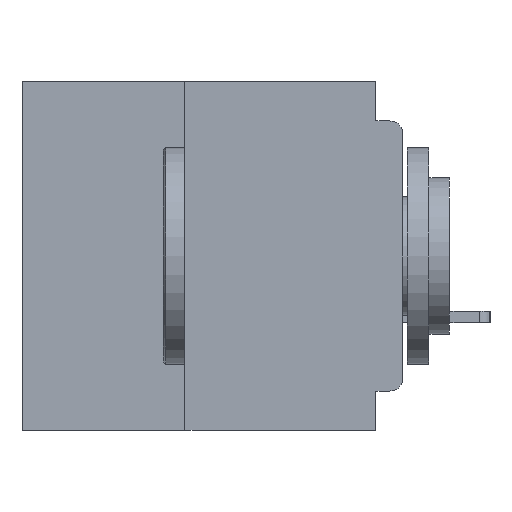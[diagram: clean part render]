
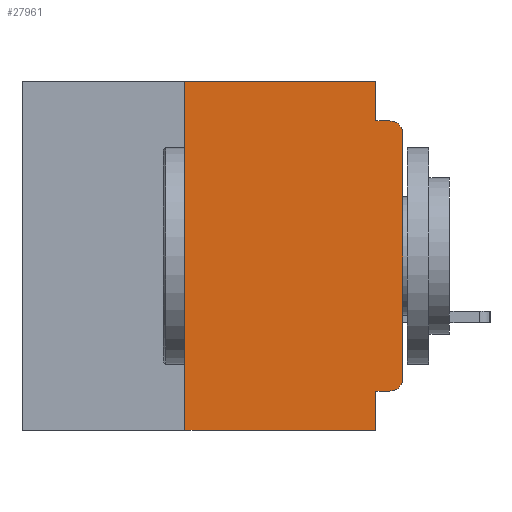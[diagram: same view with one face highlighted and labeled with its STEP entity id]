
A CAD part, left-side view. The second image highlights one B-rep face of the part: STEP entity #27961.
In plain terms, the highlighted planar face has unit normal (-1, 0, 0).
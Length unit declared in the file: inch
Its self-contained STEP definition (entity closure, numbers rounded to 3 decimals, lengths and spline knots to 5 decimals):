
#217 = ORIENTED_EDGE ( 'NONE', *, *, #29922, .F. ) ;
#635 = LINE ( 'NONE', #25883, #41856 ) ;
#734 = LINE ( 'NONE', #7674, #25898 ) ;
#1205 = DIRECTION ( 'NONE',  ( 0., -1., 0. ) ) ;
#1391 = CARTESIAN_POINT ( 'NONE',  ( 0., 0., -0.34 ) ) ;
#1689 = ORIENTED_EDGE ( 'NONE', *, *, #21981, .T. ) ;
#1900 = DIRECTION ( 'NONE',  ( 0., 0., -1. ) ) ;
#2132 = ORIENTED_EDGE ( 'NONE', *, *, #3374, .F. ) ;
#2778 = LINE ( 'NONE', #36314, #36477 ) ;
#2898 = VERTEX_POINT ( 'NONE', #15394 ) ;
#3005 = ORIENTED_EDGE ( 'NONE', *, *, #39471, .T. ) ;
#3374 = EDGE_CURVE ( 'NONE', #32404, #17091, #2778, .T. ) ;
#5257 = ORIENTED_EDGE ( 'NONE', *, *, #13119, .F. ) ;
#5487 = CARTESIAN_POINT ( 'NONE',  ( 0., 0.015, -0.355 ) ) ;
#6207 = DIRECTION ( 'NONE',  ( 0., 0., -1. ) ) ;
#6718 = VERTEX_POINT ( 'NONE', #18463 ) ;
#6780 = VECTOR ( 'NONE', #1205, 39.37008 ) ;
#7626 = CARTESIAN_POINT ( 'NONE',  ( 0., 0.031, -0.355 ) ) ;
#7674 = CARTESIAN_POINT ( 'NONE',  ( 0., 0., -0.355 ) ) ;
#7677 = VERTEX_POINT ( 'NONE', #36367 ) ;
#8104 = EDGE_CURVE ( 'NONE', #7677, #29973, #12702, .T. ) ;
#8175 = DIRECTION ( 'NONE',  ( 1., 0., 0. ) ) ;
#10160 = CIRCLE ( 'NONE', #20442, 0.015 ) ;
#10386 = VERTEX_POINT ( 'NONE', #5487 ) ;
#10614 = VECTOR ( 'NONE', #22457, 39.37008 ) ;
#10728 = VECTOR ( 'NONE', #27798, 39.37008 ) ;
#10972 = DIRECTION ( 'NONE',  ( 0., 1., 0. ) ) ;
#11464 = VERTEX_POINT ( 'NONE', #1391 ) ;
#12702 = LINE ( 'NONE', #15879, #10614 ) ;
#13119 = EDGE_CURVE ( 'NONE', #2898, #32404, #32906, .T. ) ;
#13510 = FACE_OUTER_BOUND ( 'NONE', #18480, .T. ) ;
#13540 = DIRECTION ( 'NONE',  ( 0., 0., -1. ) ) ;
#14901 = CARTESIAN_POINT ( 'NONE',  ( 0., 0.031, -0.4 ) ) ;
#14993 = LINE ( 'NONE', #24267, #31355 ) ;
#15394 = CARTESIAN_POINT ( 'NONE',  ( 0., 0.25, 0. ) ) ;
#15615 = ORIENTED_EDGE ( 'NONE', *, *, #27222, .F. ) ;
#15879 = CARTESIAN_POINT ( 'NONE',  ( 0., 0.437, -0.4 ) ) ;
#17091 = VERTEX_POINT ( 'NONE', #39140 ) ;
#17182 = LINE ( 'NONE', #21029, #24830 ) ;
#17997 = CARTESIAN_POINT ( 'NONE',  ( 0., 0.015, -0.34 ) ) ;
#18463 = CARTESIAN_POINT ( 'NONE',  ( 0., 0.015, -0.045 ) ) ;
#18480 = EDGE_LOOP ( 'NONE', ( #3005, #1689, #217, #2132, #5257, #24206, #30717, #40526, #15615, #28762 ) ) ;
#19426 = CIRCLE ( 'NONE', #24236, 0.015 ) ;
#19869 = CARTESIAN_POINT ( 'NONE',  ( 0., 0.031, 0. ) ) ;
#20442 = AXIS2_PLACEMENT_3D ( 'NONE', #17997, #40565, #21245 ) ;
#21029 = CARTESIAN_POINT ( 'NONE',  ( 0., 0.25, -0.4 ) ) ;
#21245 = DIRECTION ( 'NONE',  ( 0., 0., -1. ) ) ;
#21559 = DIRECTION ( 'NONE',  ( -1., 0., 0. ) ) ;
#21981 = EDGE_CURVE ( 'NONE', #33886, #6718, #19426, .T. ) ;
#22457 = DIRECTION ( 'NONE',  ( 0., -1., 0. ) ) ;
#22544 = EDGE_CURVE ( 'NONE', #10386, #11464, #10160, .T. ) ;
#24206 = ORIENTED_EDGE ( 'NONE', *, *, #24854, .F. ) ;
#24236 = AXIS2_PLACEMENT_3D ( 'NONE', #40893, #21559, #1900 ) ;
#24267 = CARTESIAN_POINT ( 'NONE',  ( 0., 0., 0. ) ) ;
#24469 = CARTESIAN_POINT ( 'NONE',  ( 0., 0., -0.045 ) ) ;
#24830 = VECTOR ( 'NONE', #40350, 39.37008 ) ;
#24854 = EDGE_CURVE ( 'NONE', #7677, #2898, #17182, .T. ) ;
#25883 = CARTESIAN_POINT ( 'NONE',  ( 0., 0.031, -0.4 ) ) ;
#25898 = VECTOR ( 'NONE', #10972, 39.37008 ) ;
#27222 = EDGE_CURVE ( 'NONE', #10386, #34266, #734, .T. ) ;
#27603 = DIRECTION ( 'NONE',  ( 0., 0., 1. ) ) ;
#27798 = DIRECTION ( 'NONE',  ( 0., -1., 0. ) ) ;
#27881 = PLANE ( 'NONE',  #36329 ) ;
#27961 = ADVANCED_FACE ( 'NONE', ( #13510 ), #27881, .F. ) ;
#28762 = ORIENTED_EDGE ( 'NONE', *, *, #22544, .T. ) ;
#29922 = EDGE_CURVE ( 'NONE', #17091, #6718, #36732, .T. ) ;
#29973 = VERTEX_POINT ( 'NONE', #14901 ) ;
#30717 = ORIENTED_EDGE ( 'NONE', *, *, #8104, .T. ) ;
#31149 = DIRECTION ( 'NONE',  ( 0., 0., -1. ) ) ;
#31355 = VECTOR ( 'NONE', #27603, 39.37008 ) ;
#32404 = VERTEX_POINT ( 'NONE', #19869 ) ;
#32906 = LINE ( 'NONE', #40203, #6780 ) ;
#33886 = VERTEX_POINT ( 'NONE', #37978 ) ;
#34266 = VERTEX_POINT ( 'NONE', #7626 ) ;
#36314 = CARTESIAN_POINT ( 'NONE',  ( 0., 0.031, 0. ) ) ;
#36329 = AXIS2_PLACEMENT_3D ( 'NONE', #40601, #8175, #31149 ) ;
#36367 = CARTESIAN_POINT ( 'NONE',  ( 0., 0.25, -0.4 ) ) ;
#36477 = VECTOR ( 'NONE', #13540, 39.37008 ) ;
#36732 = LINE ( 'NONE', #24469, #10728 ) ;
#37351 = EDGE_CURVE ( 'NONE', #34266, #29973, #635, .T. ) ;
#37978 = CARTESIAN_POINT ( 'NONE',  ( 0., 0., -0.06 ) ) ;
#39140 = CARTESIAN_POINT ( 'NONE',  ( 0., 0.031, -0.045 ) ) ;
#39471 = EDGE_CURVE ( 'NONE', #11464, #33886, #14993, .T. ) ;
#40203 = CARTESIAN_POINT ( 'NONE',  ( 0., 0.437, 0. ) ) ;
#40350 = DIRECTION ( 'NONE',  ( 0., 0., 1. ) ) ;
#40526 = ORIENTED_EDGE ( 'NONE', *, *, #37351, .F. ) ;
#40565 = DIRECTION ( 'NONE',  ( -1., 0., 0. ) ) ;
#40601 = CARTESIAN_POINT ( 'NONE',  ( 0., 0.437, 0. ) ) ;
#40893 = CARTESIAN_POINT ( 'NONE',  ( 0., 0.015, -0.06 ) ) ;
#41856 = VECTOR ( 'NONE', #6207, 39.37008 ) ;
